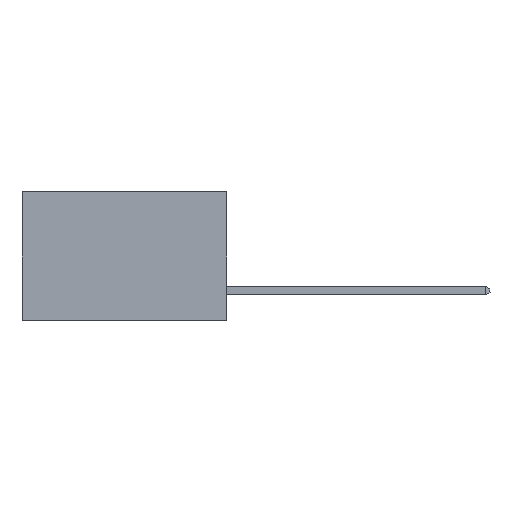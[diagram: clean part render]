
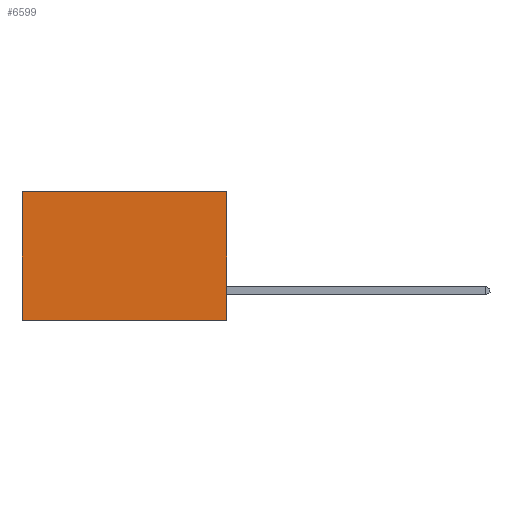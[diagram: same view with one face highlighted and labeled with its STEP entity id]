
A CAD part, left-side view. The second image highlights one B-rep face of the part: STEP entity #6599.
In plain terms, the highlighted planar face has unit normal (-1, 0, 0).
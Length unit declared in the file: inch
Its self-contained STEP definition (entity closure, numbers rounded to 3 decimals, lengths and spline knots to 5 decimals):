
#12 = CARTESIAN_POINT ( 'NONE',  ( 0.277, 0., -0.37 ) ) ;
#24 = FACE_OUTER_BOUND ( 'NONE', #13003, .T. ) ;
#394 = DIRECTION ( 'NONE',  ( 0., 1., 0. ) ) ;
#873 = VERTEX_POINT ( 'NONE', #7435 ) ;
#882 = VERTEX_POINT ( 'NONE', #1843 ) ;
#1271 = VERTEX_POINT ( 'NONE', #4376 ) ;
#1428 = EDGE_CURVE ( 'NONE', #882, #1271, #11079, .T. ) ;
#1455 = EDGE_CURVE ( 'NONE', #11799, #882, #7839, .T. ) ;
#1843 = CARTESIAN_POINT ( 'NONE',  ( 0.277, 0., -0.37 ) ) ;
#2709 = LINE ( 'NONE', #12801, #14086 ) ;
#4376 = CARTESIAN_POINT ( 'NONE',  ( 0.277, 0.59, -0.37 ) ) ;
#5425 = DIRECTION ( 'NONE',  ( 0., 0., -1. ) ) ;
#5469 = ORIENTED_EDGE ( 'NONE', *, *, #1455, .F. ) ;
#5518 = PLANE ( 'NONE',  #12595 ) ;
#5888 = EDGE_CURVE ( 'NONE', #873, #1271, #8465, .T. ) ;
#6221 = CARTESIAN_POINT ( 'NONE',  ( 0.277, 0., -0.37 ) ) ;
#6599 = ADVANCED_FACE ( 'NONE', ( #24 ), #5518, .F. ) ;
#7435 = CARTESIAN_POINT ( 'NONE',  ( 0.277, 0.59, 0. ) ) ;
#7839 = LINE ( 'NONE', #12, #13273 ) ;
#8183 = VECTOR ( 'NONE', #14502, 39.37008 ) ;
#8465 = LINE ( 'NONE', #13905, #14207 ) ;
#8864 = DIRECTION ( 'NONE',  ( 1., 0., 0. ) ) ;
#11024 = ORIENTED_EDGE ( 'NONE', *, *, #5888, .T. ) ;
#11079 = LINE ( 'NONE', #12397, #8183 ) ;
#11522 = DIRECTION ( 'NONE',  ( 0., 0., -1. ) ) ;
#11799 = VERTEX_POINT ( 'NONE', #13089 ) ;
#12397 = CARTESIAN_POINT ( 'NONE',  ( 0.277, 0., -0.37 ) ) ;
#12595 = AXIS2_PLACEMENT_3D ( 'NONE', #6221, #8864, #5425 ) ;
#12801 = CARTESIAN_POINT ( 'NONE',  ( 0.277, 0., 0. ) ) ;
#13003 = EDGE_LOOP ( 'NONE', ( #11024, #13872, #5469, #14195 ) ) ;
#13089 = CARTESIAN_POINT ( 'NONE',  ( 0.277, 0., 0. ) ) ;
#13273 = VECTOR ( 'NONE', #11522, 39.37008 ) ;
#13432 = EDGE_CURVE ( 'NONE', #11799, #873, #2709, .T. ) ;
#13864 = DIRECTION ( 'NONE',  ( 0., 0., -1. ) ) ;
#13872 = ORIENTED_EDGE ( 'NONE', *, *, #1428, .F. ) ;
#13905 = CARTESIAN_POINT ( 'NONE',  ( 0.277, 0.59, -0.37 ) ) ;
#14086 = VECTOR ( 'NONE', #394, 39.37008 ) ;
#14195 = ORIENTED_EDGE ( 'NONE', *, *, #13432, .T. ) ;
#14207 = VECTOR ( 'NONE', #13864, 39.37008 ) ;
#14502 = DIRECTION ( 'NONE',  ( 0., 1., 0. ) ) ;
